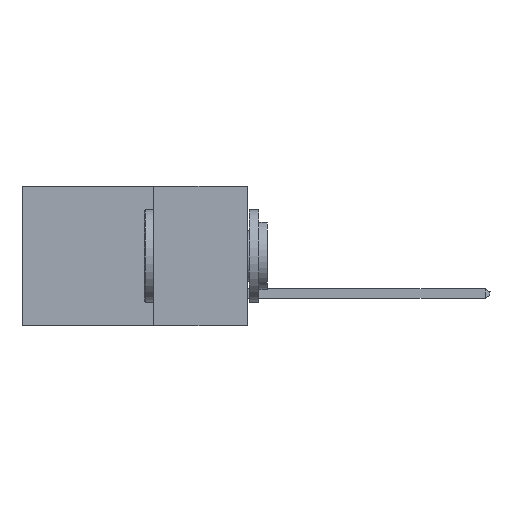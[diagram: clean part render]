
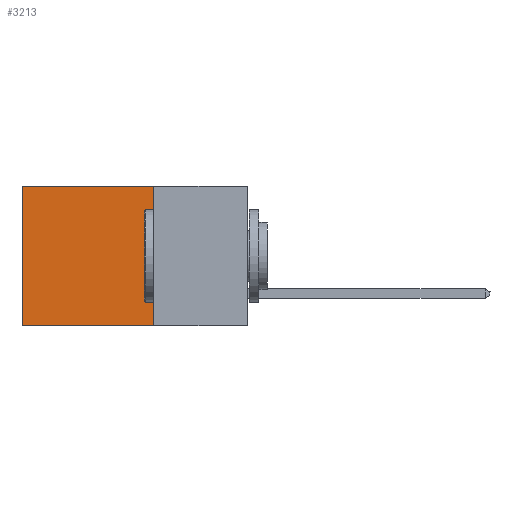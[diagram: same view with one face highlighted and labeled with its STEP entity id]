
A CAD part, left-side view. The second image highlights one B-rep face of the part: STEP entity #3213.
In plain terms, the highlighted planar face has unit normal (-1, 0, 0).
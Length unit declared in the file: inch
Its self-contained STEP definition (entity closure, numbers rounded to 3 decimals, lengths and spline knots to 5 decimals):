
#149 = CARTESIAN_POINT ( 'NONE',  ( 0.2615, 0.6, -0.37 ) ) ;
#178 = EDGE_CURVE ( 'NONE', #8649, #10419, #15444, .T. ) ;
#232 = AXIS2_PLACEMENT_3D ( 'NONE', #3222, #5607, #14315 ) ;
#350 = LINE ( 'NONE', #14983, #698 ) ;
#698 = VECTOR ( 'NONE', #2735, 39.37008 ) ;
#1141 = VERTEX_POINT ( 'NONE', #5893 ) ;
#1437 = EDGE_CURVE ( 'NONE', #10419, #14687, #5454, .T. ) ;
#2173 = ORIENTED_EDGE ( 'NONE', *, *, #5801, .T. ) ;
#2735 = DIRECTION ( 'NONE',  ( 0., 0., -1. ) ) ;
#2746 = DIRECTION ( 'NONE',  ( 0., 1., 0. ) ) ;
#2854 = CARTESIAN_POINT ( 'NONE',  ( 0.2615, 0.25, 0. ) ) ;
#3213 = ADVANCED_FACE ( 'NONE', ( #4694 ), #9626, .F. ) ;
#3222 = CARTESIAN_POINT ( 'NONE',  ( 0.2615, 0.25, -0.37 ) ) ;
#4694 = FACE_OUTER_BOUND ( 'NONE', #13342, .T. ) ;
#5291 = ORIENTED_EDGE ( 'NONE', *, *, #1437, .F. ) ;
#5454 = LINE ( 'NONE', #6438, #12368 ) ;
#5607 = DIRECTION ( 'NONE',  ( 1., 0., 0. ) ) ;
#5728 = VECTOR ( 'NONE', #12862, 39.37008 ) ;
#5801 = EDGE_CURVE ( 'NONE', #8649, #1141, #12614, .T. ) ;
#5893 = CARTESIAN_POINT ( 'NONE',  ( 0.2615, 0.6, 0. ) ) ;
#5932 = ORIENTED_EDGE ( 'NONE', *, *, #178, .F. ) ;
#6438 = CARTESIAN_POINT ( 'NONE',  ( 0.2615, 0.25, -0.37 ) ) ;
#6610 = EDGE_CURVE ( 'NONE', #1141, #14687, #350, .T. ) ;
#7574 = ORIENTED_EDGE ( 'NONE', *, *, #6610, .T. ) ;
#7975 = CARTESIAN_POINT ( 'NONE',  ( 0.2615, 0.25, -0.37 ) ) ;
#8649 = VERTEX_POINT ( 'NONE', #2854 ) ;
#9580 = CARTESIAN_POINT ( 'NONE',  ( 0.2615, 0.25, -0.37 ) ) ;
#9626 = PLANE ( 'NONE',  #232 ) ;
#10419 = VERTEX_POINT ( 'NONE', #9580 ) ;
#12368 = VECTOR ( 'NONE', #2746, 39.37008 ) ;
#12614 = LINE ( 'NONE', #13855, #5728 ) ;
#12862 = DIRECTION ( 'NONE',  ( 0., 1., 0. ) ) ;
#13222 = DIRECTION ( 'NONE',  ( 0., 0., -1. ) ) ;
#13342 = EDGE_LOOP ( 'NONE', ( #7574, #5291, #5932, #2173 ) ) ;
#13707 = VECTOR ( 'NONE', #13222, 39.37008 ) ;
#13855 = CARTESIAN_POINT ( 'NONE',  ( 0.2615, 0.25, 0. ) ) ;
#14315 = DIRECTION ( 'NONE',  ( 0., 0., -1. ) ) ;
#14687 = VERTEX_POINT ( 'NONE', #149 ) ;
#14983 = CARTESIAN_POINT ( 'NONE',  ( 0.2615, 0.6, -0.37 ) ) ;
#15444 = LINE ( 'NONE', #7975, #13707 ) ;
